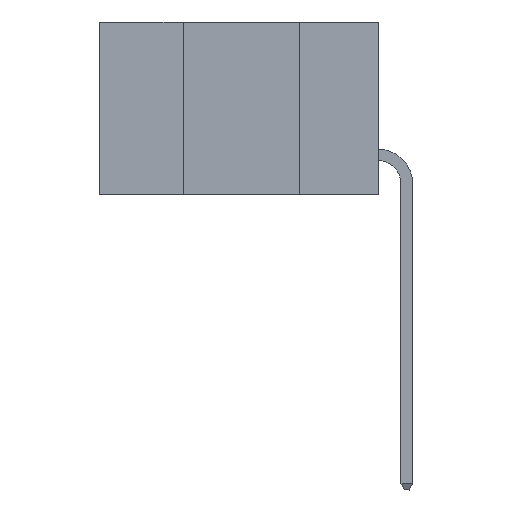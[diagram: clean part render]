
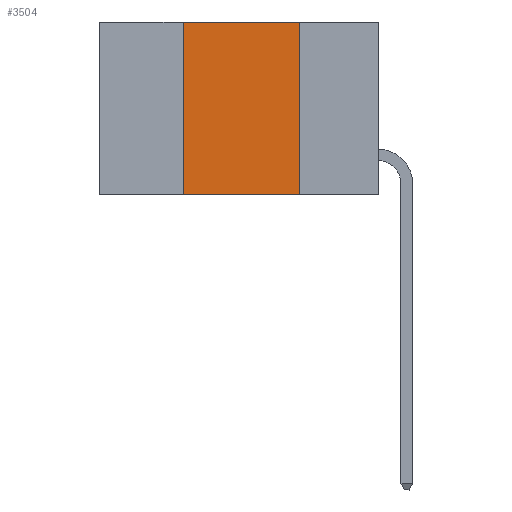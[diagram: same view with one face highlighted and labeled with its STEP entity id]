
A CAD part, left-side view. The second image highlights one B-rep face of the part: STEP entity #3504.
In plain terms, the highlighted planar face has unit normal (-1, 0, 0).
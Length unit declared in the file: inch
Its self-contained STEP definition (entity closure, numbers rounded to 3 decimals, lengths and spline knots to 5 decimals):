
#284 = CARTESIAN_POINT ( 'NONE',  ( 0., 0.17, -0.37 ) ) ;
#412 = VERTEX_POINT ( 'NONE', #1413 ) ;
#539 = CARTESIAN_POINT ( 'NONE',  ( 0., 0.6, -0.37 ) ) ;
#1413 = CARTESIAN_POINT ( 'NONE',  ( 0., 0.17, 0. ) ) ;
#1858 = ORIENTED_EDGE ( 'NONE', *, *, #17392, .F. ) ;
#2085 = LINE ( 'NONE', #284, #7170 ) ;
#2230 = DIRECTION ( 'NONE',  ( 0., -1., 0. ) ) ;
#3504 = ADVANCED_FACE ( 'NONE', ( #9839 ), #20783, .F. ) ;
#3679 = DIRECTION ( 'NONE',  ( 0., 0., -1. ) ) ;
#6101 = EDGE_CURVE ( 'NONE', #6278, #13295, #10043, .T. ) ;
#6278 = VERTEX_POINT ( 'NONE', #7715 ) ;
#6992 = AXIS2_PLACEMENT_3D ( 'NONE', #8261, #7843, #14250 ) ;
#7071 = EDGE_CURVE ( 'NONE', #15509, #412, #13126, .T. ) ;
#7170 = VECTOR ( 'NONE', #3679, 39.37008 ) ;
#7218 = CARTESIAN_POINT ( 'NONE',  ( 0., 0.42, -0.37 ) ) ;
#7715 = CARTESIAN_POINT ( 'NONE',  ( 0., 0.42, -0.37 ) ) ;
#7843 = DIRECTION ( 'NONE',  ( 1., 0., 0. ) ) ;
#8261 = CARTESIAN_POINT ( 'NONE',  ( 0., 0.6, 0. ) ) ;
#8502 = VECTOR ( 'NONE', #14808, 39.37008 ) ;
#9839 = FACE_OUTER_BOUND ( 'NONE', #19173, .T. ) ;
#9999 = CARTESIAN_POINT ( 'NONE',  ( 0., 0.6, 0. ) ) ;
#10043 = LINE ( 'NONE', #539, #17173 ) ;
#10647 = ORIENTED_EDGE ( 'NONE', *, *, #10877, .F. ) ;
#10877 = EDGE_CURVE ( 'NONE', #6278, #15509, #18371, .T. ) ;
#12606 = ORIENTED_EDGE ( 'NONE', *, *, #6101, .T. ) ;
#13126 = LINE ( 'NONE', #9999, #8502 ) ;
#13295 = VERTEX_POINT ( 'NONE', #16455 ) ;
#13937 = DIRECTION ( 'NONE',  ( 0., 0., 1. ) ) ;
#14129 = VECTOR ( 'NONE', #13937, 39.37008 ) ;
#14250 = DIRECTION ( 'NONE',  ( 0., 0., -1. ) ) ;
#14808 = DIRECTION ( 'NONE',  ( 0., -1., 0. ) ) ;
#15509 = VERTEX_POINT ( 'NONE', #17759 ) ;
#16455 = CARTESIAN_POINT ( 'NONE',  ( 0., 0.17, -0.37 ) ) ;
#17173 = VECTOR ( 'NONE', #2230, 39.37008 ) ;
#17392 = EDGE_CURVE ( 'NONE', #412, #13295, #2085, .T. ) ;
#17759 = CARTESIAN_POINT ( 'NONE',  ( 0., 0.42, 0. ) ) ;
#18371 = LINE ( 'NONE', #7218, #14129 ) ;
#19173 = EDGE_LOOP ( 'NONE', ( #1858, #20680, #10647, #12606 ) ) ;
#20680 = ORIENTED_EDGE ( 'NONE', *, *, #7071, .F. ) ;
#20783 = PLANE ( 'NONE',  #6992 ) ;
